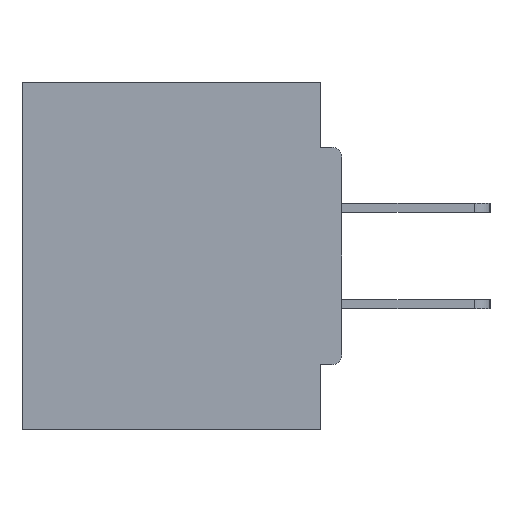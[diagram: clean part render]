
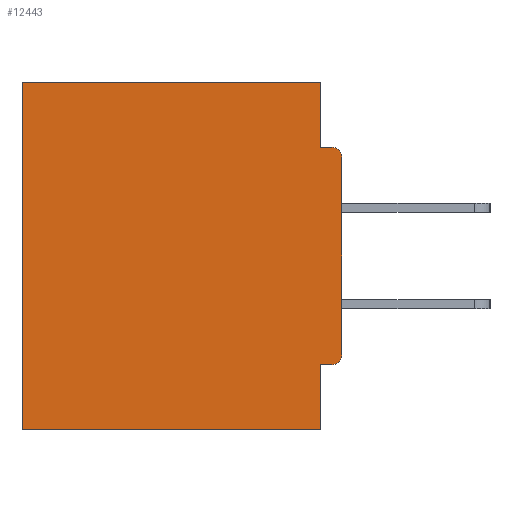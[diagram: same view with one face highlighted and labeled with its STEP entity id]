
A CAD part, left-side view. The second image highlights one B-rep face of the part: STEP entity #12443.
In plain terms, the highlighted planar face has unit normal (-1, 0, 0).
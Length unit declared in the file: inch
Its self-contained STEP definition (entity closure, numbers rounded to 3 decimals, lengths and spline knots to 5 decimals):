
#18 = EDGE_CURVE ( 'NONE', #26798, #6196, #24058, .T. ) ;
#151 = LINE ( 'NONE', #9811, #24729 ) ;
#268 = PLANE ( 'NONE',  #7920 ) ;
#393 = EDGE_CURVE ( 'NONE', #22243, #32969, #13198, .T. ) ;
#571 = DIRECTION ( 'NONE',  ( -1., 0., 0. ) ) ;
#651 = ORIENTED_EDGE ( 'NONE', *, *, #25745, .F. ) ;
#1419 = EDGE_CURVE ( 'NONE', #29984, #22243, #6709, .T. ) ;
#1469 = ORIENTED_EDGE ( 'NONE', *, *, #1419, .T. ) ;
#1640 = ORIENTED_EDGE ( 'NONE', *, *, #5641, .F. ) ;
#1834 = AXIS2_PLACEMENT_3D ( 'NONE', #11418, #21929, #29978 ) ;
#2682 = VERTEX_POINT ( 'NONE', #34218 ) ;
#3980 = CARTESIAN_POINT ( 'NONE',  ( 0.298, 0., -0.1085 ) ) ;
#4220 = CARTESIAN_POINT ( 'NONE',  ( 0.298, 0.031, -0.5 ) ) ;
#5359 = CARTESIAN_POINT ( 'NONE',  ( 0.298, 0.46, 0. ) ) ;
#5641 = EDGE_CURVE ( 'NONE', #30243, #34355, #151, .T. ) ;
#5773 = LINE ( 'NONE', #4220, #15740 ) ;
#6196 = VERTEX_POINT ( 'NONE', #16276 ) ;
#6293 = CARTESIAN_POINT ( 'NONE',  ( 0.298, 0.015, -0.3915 ) ) ;
#6709 = LINE ( 'NONE', #7186, #13340 ) ;
#6763 = CARTESIAN_POINT ( 'NONE',  ( 0.298, 0.031, -0.4065 ) ) ;
#7086 = ORIENTED_EDGE ( 'NONE', *, *, #29912, .F. ) ;
#7186 = CARTESIAN_POINT ( 'NONE',  ( 0.298, 0., 0. ) ) ;
#7432 = CARTESIAN_POINT ( 'NONE',  ( 0.298, 0.46, 0. ) ) ;
#7858 = VERTEX_POINT ( 'NONE', #25853 ) ;
#7920 = AXIS2_PLACEMENT_3D ( 'NONE', #18791, #18899, #16092 ) ;
#8594 = CARTESIAN_POINT ( 'NONE',  ( 0.298, 0.46, -0.5 ) ) ;
#9197 = FACE_OUTER_BOUND ( 'NONE', #23259, .T. ) ;
#9459 = CIRCLE ( 'NONE', #1834, 0.015 ) ;
#9811 = CARTESIAN_POINT ( 'NONE',  ( 0.298, 0., -0.4065 ) ) ;
#9897 = VECTOR ( 'NONE', #14072, 39.37008 ) ;
#11382 = CARTESIAN_POINT ( 'NONE',  ( 0.298, 0., 0. ) ) ;
#11418 = CARTESIAN_POINT ( 'NONE',  ( 0.298, 0.015, -0.1085 ) ) ;
#12443 = ADVANCED_FACE ( 'NONE', ( #9197 ), #268, .F. ) ;
#13146 = CARTESIAN_POINT ( 'NONE',  ( 0.298, 0.015, -0.4065 ) ) ;
#13198 = LINE ( 'NONE', #7432, #19456 ) ;
#13340 = VECTOR ( 'NONE', #34405, 39.37008 ) ;
#13623 = LINE ( 'NONE', #24376, #34045 ) ;
#13874 = ORIENTED_EDGE ( 'NONE', *, *, #393, .T. ) ;
#14016 = DIRECTION ( 'NONE',  ( 0., -1., 0. ) ) ;
#14072 = DIRECTION ( 'NONE',  ( 0., 0., -1. ) ) ;
#14310 = LINE ( 'NONE', #30651, #25961 ) ;
#15344 = EDGE_CURVE ( 'NONE', #7858, #32969, #25388, .T. ) ;
#15740 = VECTOR ( 'NONE', #30768, 39.37008 ) ;
#16092 = DIRECTION ( 'NONE',  ( 0., 0., -1. ) ) ;
#16224 = CARTESIAN_POINT ( 'NONE',  ( 0.298, 0.031, -0.0935 ) ) ;
#16276 = CARTESIAN_POINT ( 'NONE',  ( 0.298, 0., -0.3915 ) ) ;
#16820 = ORIENTED_EDGE ( 'NONE', *, *, #15344, .F. ) ;
#17353 = CARTESIAN_POINT ( 'NONE',  ( 0.298, 0.031, 0. ) ) ;
#17715 = DIRECTION ( 'NONE',  ( 0., 0., -1. ) ) ;
#18244 = DIRECTION ( 'NONE',  ( 0., 0., -1. ) ) ;
#18323 = VECTOR ( 'NONE', #20060, 39.37008 ) ;
#18791 = CARTESIAN_POINT ( 'NONE',  ( 0.298, 0., 0. ) ) ;
#18899 = DIRECTION ( 'NONE',  ( 1., 0., 0. ) ) ;
#19331 = DIRECTION ( 'NONE',  ( 0., 0., -1. ) ) ;
#19456 = VECTOR ( 'NONE', #18244, 39.37008 ) ;
#20060 = DIRECTION ( 'NONE',  ( 0., 1., 0. ) ) ;
#20489 = CIRCLE ( 'NONE', #21936, 0.015 ) ;
#21191 = EDGE_CURVE ( 'NONE', #30243, #6196, #20489, .T. ) ;
#21523 = VERTEX_POINT ( 'NONE', #16224 ) ;
#21929 = DIRECTION ( 'NONE',  ( -1., 0., 0. ) ) ;
#21936 = AXIS2_PLACEMENT_3D ( 'NONE', #6293, #571, #19331 ) ;
#22243 = VERTEX_POINT ( 'NONE', #5359 ) ;
#23045 = ORIENTED_EDGE ( 'NONE', *, *, #21191, .T. ) ;
#23259 = EDGE_LOOP ( 'NONE', ( #28107, #27875, #7086, #1469, #13874, #16820, #651, #1640, #23045, #32680 ) ) ;
#24058 = LINE ( 'NONE', #11382, #9897 ) ;
#24376 = CARTESIAN_POINT ( 'NONE',  ( 0.298, 0., -0.0935 ) ) ;
#24729 = VECTOR ( 'NONE', #25520, 39.37008 ) ;
#25388 = LINE ( 'NONE', #33431, #18323 ) ;
#25520 = DIRECTION ( 'NONE',  ( 0., 1., 0. ) ) ;
#25745 = EDGE_CURVE ( 'NONE', #34355, #7858, #14310, .T. ) ;
#25853 = CARTESIAN_POINT ( 'NONE',  ( 0.298, 0.031, -0.5 ) ) ;
#25961 = VECTOR ( 'NONE', #17715, 39.37008 ) ;
#26798 = VERTEX_POINT ( 'NONE', #3980 ) ;
#27875 = ORIENTED_EDGE ( 'NONE', *, *, #33455, .F. ) ;
#28107 = ORIENTED_EDGE ( 'NONE', *, *, #31590, .T. ) ;
#29912 = EDGE_CURVE ( 'NONE', #29984, #21523, #5773, .T. ) ;
#29978 = DIRECTION ( 'NONE',  ( 0., 0., -1. ) ) ;
#29984 = VERTEX_POINT ( 'NONE', #17353 ) ;
#30243 = VERTEX_POINT ( 'NONE', #13146 ) ;
#30651 = CARTESIAN_POINT ( 'NONE',  ( 0.298, 0.031, -0.5 ) ) ;
#30768 = DIRECTION ( 'NONE',  ( 0., 0., -1. ) ) ;
#31590 = EDGE_CURVE ( 'NONE', #26798, #2682, #9459, .T. ) ;
#32680 = ORIENTED_EDGE ( 'NONE', *, *, #18, .F. ) ;
#32969 = VERTEX_POINT ( 'NONE', #8594 ) ;
#33431 = CARTESIAN_POINT ( 'NONE',  ( 0.298, 0., -0.5 ) ) ;
#33455 = EDGE_CURVE ( 'NONE', #21523, #2682, #13623, .T. ) ;
#34045 = VECTOR ( 'NONE', #14016, 39.37008 ) ;
#34218 = CARTESIAN_POINT ( 'NONE',  ( 0.298, 0.015, -0.0935 ) ) ;
#34355 = VERTEX_POINT ( 'NONE', #6763 ) ;
#34405 = DIRECTION ( 'NONE',  ( 0., 1., 0. ) ) ;
